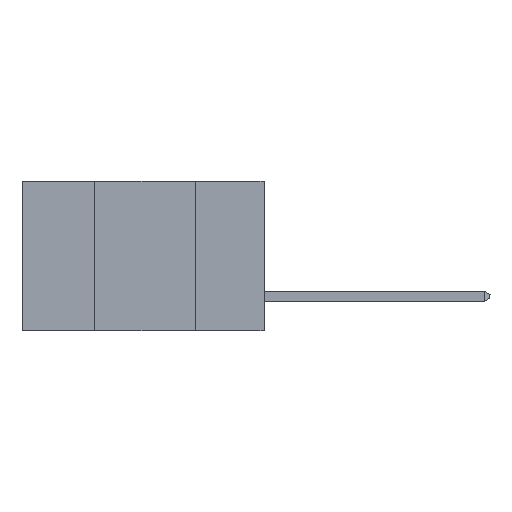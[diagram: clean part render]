
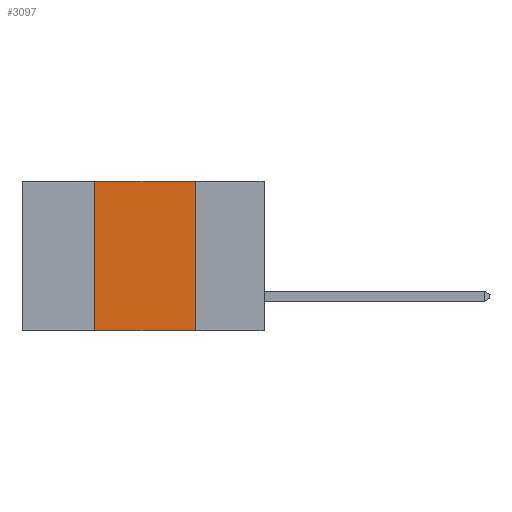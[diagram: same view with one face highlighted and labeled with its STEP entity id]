
A CAD part, left-side view. The second image highlights one B-rep face of the part: STEP entity #3097.
In plain terms, the highlighted planar face has unit normal (-1, 0, 0).
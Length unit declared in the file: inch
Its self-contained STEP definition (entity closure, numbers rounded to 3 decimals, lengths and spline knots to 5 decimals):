
#163 = DIRECTION ( 'NONE',  ( 0., 0., -1. ) ) ;
#379 = CARTESIAN_POINT ( 'NONE',  ( 0., 0.6, -0.37 ) ) ;
#661 = CARTESIAN_POINT ( 'NONE',  ( 0., 0.17, -0.37 ) ) ;
#705 = CARTESIAN_POINT ( 'NONE',  ( 0., 0.42, -0.37 ) ) ;
#721 = VECTOR ( 'NONE', #3630, 39.37008 ) ;
#884 = FACE_OUTER_BOUND ( 'NONE', #7118, .T. ) ;
#1228 = CARTESIAN_POINT ( 'NONE',  ( 0., 0.17, -0.37 ) ) ;
#1435 = LINE ( 'NONE', #1485, #6610 ) ;
#1485 = CARTESIAN_POINT ( 'NONE',  ( 0., 0.42, -0.37 ) ) ;
#1596 = VECTOR ( 'NONE', #163, 39.37008 ) ;
#1809 = CARTESIAN_POINT ( 'NONE',  ( 0., 0.6, 0. ) ) ;
#2518 = DIRECTION ( 'NONE',  ( 1., 0., 0. ) ) ;
#2537 = LINE ( 'NONE', #661, #1596 ) ;
#2559 = EDGE_CURVE ( 'NONE', #5112, #7882, #1435, .T. ) ;
#2651 = LINE ( 'NONE', #1809, #6884 ) ;
#3097 = ADVANCED_FACE ( 'NONE', ( #884 ), #4825, .F. ) ;
#3565 = DIRECTION ( 'NONE',  ( 0., -1., 0. ) ) ;
#3630 = DIRECTION ( 'NONE',  ( 0., -1., 0. ) ) ;
#4142 = EDGE_CURVE ( 'NONE', #5112, #8357, #6798, .T. ) ;
#4825 = PLANE ( 'NONE',  #9220 ) ;
#4882 = DIRECTION ( 'NONE',  ( 0., 0., -1. ) ) ;
#5112 = VERTEX_POINT ( 'NONE', #705 ) ;
#5845 = EDGE_CURVE ( 'NONE', #7882, #7661, #2651, .T. ) ;
#5944 = ORIENTED_EDGE ( 'NONE', *, *, #9777, .F. ) ;
#6610 = VECTOR ( 'NONE', #7836, 39.37008 ) ;
#6798 = LINE ( 'NONE', #379, #721 ) ;
#6884 = VECTOR ( 'NONE', #3565, 39.37008 ) ;
#6895 = ORIENTED_EDGE ( 'NONE', *, *, #4142, .T. ) ;
#7118 = EDGE_LOOP ( 'NONE', ( #5944, #8862, #8173, #6895 ) ) ;
#7239 = CARTESIAN_POINT ( 'NONE',  ( 0., 0.6, 0. ) ) ;
#7661 = VERTEX_POINT ( 'NONE', #7880 ) ;
#7836 = DIRECTION ( 'NONE',  ( 0., 0., 1. ) ) ;
#7880 = CARTESIAN_POINT ( 'NONE',  ( 0., 0.17, 0. ) ) ;
#7882 = VERTEX_POINT ( 'NONE', #9306 ) ;
#8173 = ORIENTED_EDGE ( 'NONE', *, *, #2559, .F. ) ;
#8357 = VERTEX_POINT ( 'NONE', #1228 ) ;
#8862 = ORIENTED_EDGE ( 'NONE', *, *, #5845, .F. ) ;
#9220 = AXIS2_PLACEMENT_3D ( 'NONE', #7239, #2518, #4882 ) ;
#9306 = CARTESIAN_POINT ( 'NONE',  ( 0., 0.42, 0. ) ) ;
#9777 = EDGE_CURVE ( 'NONE', #7661, #8357, #2537, .T. ) ;
